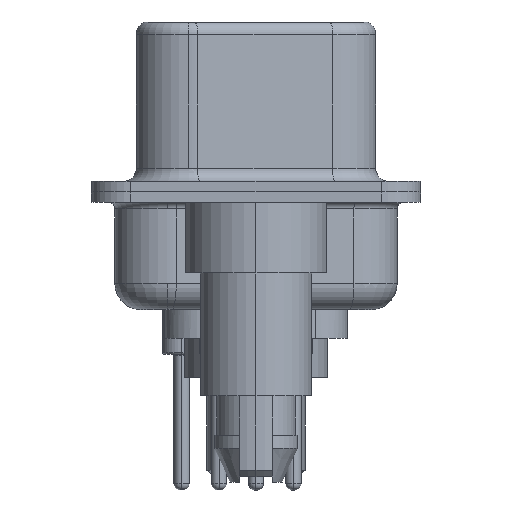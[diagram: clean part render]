
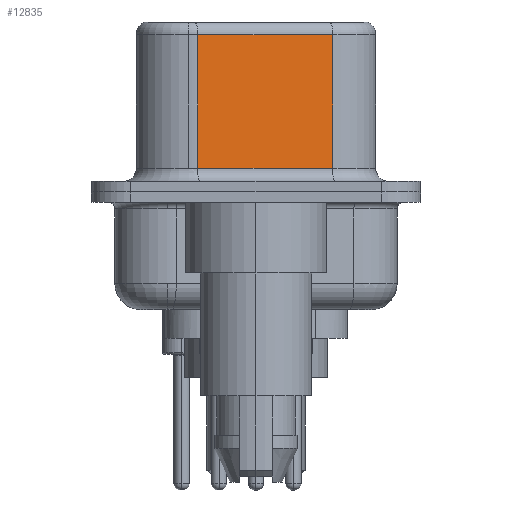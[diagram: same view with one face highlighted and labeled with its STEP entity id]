
A CAD part, left-side view. The second image highlights one B-rep face of the part: STEP entity #12835.
In plain terms, the highlighted planar face has unit normal (-0.985, -0.174, 0).
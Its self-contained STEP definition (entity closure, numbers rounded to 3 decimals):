
#99 = FACE_OUTER_BOUND ( 'NONE', #22593, .T. ) ;
#379 = CARTESIAN_POINT ( 'NONE',  ( 3.675, 2.233, 6.02 ) ) ;
#822 = VECTOR ( 'NONE', #5744, 1000. ) ;
#1096 = CARTESIAN_POINT ( 'NONE',  ( 4.585, -2.927, 6.52 ) ) ;
#1616 = EDGE_CURVE ( 'NONE', #19008, #4434, #20382, .T. ) ;
#2730 = LINE ( 'NONE', #17592, #822 ) ;
#3883 = VECTOR ( 'NONE', #21242, 1000. ) ;
#4434 = VERTEX_POINT ( 'NONE', #20515 ) ;
#4904 = DIRECTION ( 'NONE',  ( -0.174, 0.985, 0. ) ) ;
#5744 = DIRECTION ( 'NONE',  ( 0., 0., -1. ) ) ;
#10093 = CARTESIAN_POINT ( 'NONE',  ( 4.585, -2.927, 6.02 ) ) ;
#12014 = DIRECTION ( 'NONE',  ( 0., 0., -1. ) ) ;
#12059 = VECTOR ( 'NONE', #12014, 1000. ) ;
#12143 = EDGE_CURVE ( 'NONE', #19008, #22355, #22471, .T. ) ;
#12694 = PLANE ( 'NONE',  #25093 ) ;
#12731 = ORIENTED_EDGE ( 'NONE', *, *, #22527, .T. ) ;
#12835 = ADVANCED_FACE ( 'NONE', ( #99 ), #12694, .F. ) ;
#13385 = CARTESIAN_POINT ( 'NONE',  ( 4.585, -2.927, 0.9 ) ) ;
#14184 = CARTESIAN_POINT ( 'NONE',  ( 4.585, -2.927, 6.02 ) ) ;
#15695 = ORIENTED_EDGE ( 'NONE', *, *, #24803, .T. ) ;
#16670 = CARTESIAN_POINT ( 'NONE',  ( 4.585, -2.927, 6.52 ) ) ;
#16965 = ORIENTED_EDGE ( 'NONE', *, *, #12143, .T. ) ;
#17006 = DIRECTION ( 'NONE',  ( 0.985, 0.174, 0. ) ) ;
#17592 = CARTESIAN_POINT ( 'NONE',  ( 3.675, 2.233, 6.52 ) ) ;
#18632 = CARTESIAN_POINT ( 'NONE',  ( 3.675, 2.233, 0.9 ) ) ;
#19008 = VERTEX_POINT ( 'NONE', #14184 ) ;
#19983 = DIRECTION ( 'NONE',  ( -0.174, 0.985, 0. ) ) ;
#20382 = LINE ( 'NONE', #1096, #12059 ) ;
#20515 = CARTESIAN_POINT ( 'NONE',  ( 4.585, -2.927, 0.9 ) ) ;
#20611 = LINE ( 'NONE', #13385, #3883 ) ;
#21242 = DIRECTION ( 'NONE',  ( 0.174, -0.985, 0. ) ) ;
#22355 = VERTEX_POINT ( 'NONE', #379 ) ;
#22471 = LINE ( 'NONE', #10093, #23698 ) ;
#22527 = EDGE_CURVE ( 'NONE', #22355, #24054, #2730, .T. ) ;
#22593 = EDGE_LOOP ( 'NONE', ( #23051, #16965, #12731, #15695 ) ) ;
#23051 = ORIENTED_EDGE ( 'NONE', *, *, #1616, .F. ) ;
#23698 = VECTOR ( 'NONE', #19983, 1000. ) ;
#24054 = VERTEX_POINT ( 'NONE', #18632 ) ;
#24803 = EDGE_CURVE ( 'NONE', #24054, #4434, #20611, .T. ) ;
#25093 = AXIS2_PLACEMENT_3D ( 'NONE', #16670, #17006, #4904 ) ;
